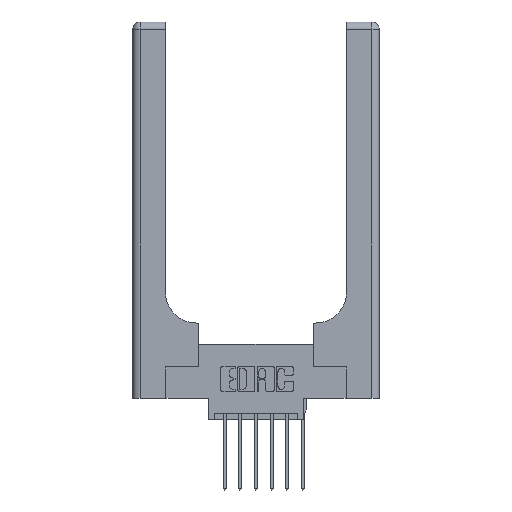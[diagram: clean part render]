
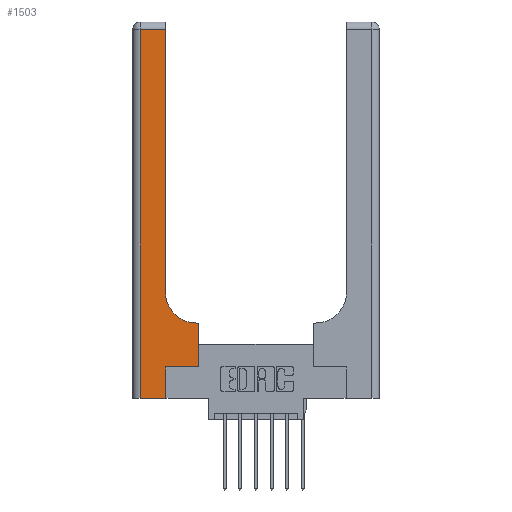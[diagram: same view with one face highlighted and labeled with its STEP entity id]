
A CAD part, top view. The second image highlights one B-rep face of the part: STEP entity #1503.
In plain terms, the highlighted planar face has unit normal (0, 0, 1).
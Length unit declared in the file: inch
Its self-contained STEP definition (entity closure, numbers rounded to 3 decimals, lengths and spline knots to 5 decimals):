
#176 = CARTESIAN_POINT ( 'NONE',  ( 0.26, 0.85, 0.37 ) ) ;
#266 = VECTOR ( 'NONE', #6925, 39.37008 ) ;
#312 = VERTEX_POINT ( 'NONE', #5157 ) ;
#846 = VERTEX_POINT ( 'NONE', #11855 ) ;
#978 = ORIENTED_EDGE ( 'NONE', *, *, #5682, .T. ) ;
#1276 = EDGE_CURVE ( 'NONE', #13701, #12622, #11691, .T. ) ;
#1503 = ADVANCED_FACE ( 'NONE', ( #12878 ), #13950, .F. ) ;
#1708 = DIRECTION ( 'NONE',  ( 1., 0., 0. ) ) ;
#1750 = CIRCLE ( 'NONE', #13360, 0.25 ) ;
#1957 = ORIENTED_EDGE ( 'NONE', *, *, #6541, .T. ) ;
#2016 = CARTESIAN_POINT ( 'NONE',  ( 0.528, 0.25, 0.37 ) ) ;
#2044 = EDGE_CURVE ( 'NONE', #2976, #13701, #1750, .T. ) ;
#2115 = DIRECTION ( 'NONE',  ( -1., 0., 0. ) ) ;
#2976 = VERTEX_POINT ( 'NONE', #3687 ) ;
#3017 = ORIENTED_EDGE ( 'NONE', *, *, #1276, .T. ) ;
#3202 = VECTOR ( 'NONE', #13751, 39.37008 ) ;
#3293 = VERTEX_POINT ( 'NONE', #9776 ) ;
#3356 = DIRECTION ( 'NONE',  ( 1., 0., 0. ) ) ;
#3436 = EDGE_CURVE ( 'NONE', #846, #3293, #11443, .T. ) ;
#3687 = CARTESIAN_POINT ( 'NONE',  ( 0.51, 0.6, 0.37 ) ) ;
#3772 = ORIENTED_EDGE ( 'NONE', *, *, #5378, .T. ) ;
#4036 = EDGE_CURVE ( 'NONE', #3293, #9507, #4855, .T. ) ;
#4099 = DIRECTION ( 'NONE',  ( 1., 0., 0. ) ) ;
#4250 = ORIENTED_EDGE ( 'NONE', *, *, #11842, .T. ) ;
#4713 = LINE ( 'NONE', #5875, #266 ) ;
#4855 = LINE ( 'NONE', #8960, #10240 ) ;
#5157 = CARTESIAN_POINT ( 'NONE',  ( 0.528, 0.25, 0.37 ) ) ;
#5203 = ORIENTED_EDGE ( 'NONE', *, *, #4036, .T. ) ;
#5378 = EDGE_CURVE ( 'NONE', #6536, #2976, #9493, .T. ) ;
#5486 = ORIENTED_EDGE ( 'NONE', *, *, #3436, .T. ) ;
#5620 = EDGE_LOOP ( 'NONE', ( #3017, #978, #13871, #5486, #5203, #1957, #4250, #3772, #9797 ) ) ;
#5682 = EDGE_CURVE ( 'NONE', #12622, #10782, #6336, .T. ) ;
#5688 = VECTOR ( 'NONE', #4099, 39.37008 ) ;
#5775 = DIRECTION ( 'NONE',  ( 0., 1., 0. ) ) ;
#5875 = CARTESIAN_POINT ( 'NONE',  ( 0.06, 3., 0.37 ) ) ;
#6336 = LINE ( 'NONE', #11702, #10401 ) ;
#6536 = VERTEX_POINT ( 'NONE', #13755 ) ;
#6541 = EDGE_CURVE ( 'NONE', #9507, #312, #10551, .T. ) ;
#6819 = VECTOR ( 'NONE', #1708, 39.37008 ) ;
#6925 = DIRECTION ( 'NONE',  ( 0., -1., 0. ) ) ;
#6979 = VECTOR ( 'NONE', #12642, 39.37008 ) ;
#6985 = VECTOR ( 'NONE', #8204, 39.37008 ) ;
#7169 = EDGE_CURVE ( 'NONE', #10782, #846, #4713, .T. ) ;
#7227 = CARTESIAN_POINT ( 'NONE',  ( 0.26, 0.6, 0.37 ) ) ;
#8204 = DIRECTION ( 'NONE',  ( 0., 1., 0. ) ) ;
#8292 = LINE ( 'NONE', #2016, #6979 ) ;
#8744 = CARTESIAN_POINT ( 'NONE',  ( 0.51, 0.85, 0.37 ) ) ;
#8960 = CARTESIAN_POINT ( 'NONE',  ( 0.265, 0., 0.37 ) ) ;
#9493 = LINE ( 'NONE', #7227, #3202 ) ;
#9507 = VERTEX_POINT ( 'NONE', #12911 ) ;
#9594 = CARTESIAN_POINT ( 'NONE',  ( 0.26, 3., 0.37 ) ) ;
#9776 = CARTESIAN_POINT ( 'NONE',  ( 0.265, 0., 0.37 ) ) ;
#9797 = ORIENTED_EDGE ( 'NONE', *, *, #2044, .T. ) ;
#10240 = VECTOR ( 'NONE', #5775, 39.37008 ) ;
#10401 = VECTOR ( 'NONE', #2115, 39.37008 ) ;
#10551 = LINE ( 'NONE', #11819, #5688 ) ;
#10782 = VERTEX_POINT ( 'NONE', #11830 ) ;
#11442 = CARTESIAN_POINT ( 'NONE',  ( 0.26, 2.94, 0.37 ) ) ;
#11443 = LINE ( 'NONE', #11508, #6819 ) ;
#11508 = CARTESIAN_POINT ( 'NONE',  ( 0., 0., 0.37 ) ) ;
#11691 = LINE ( 'NONE', #9594, #6985 ) ;
#11702 = CARTESIAN_POINT ( 'NONE',  ( 0., 2.94, 0.37 ) ) ;
#11795 = CARTESIAN_POINT ( 'NONE',  ( 0., 3., 0.37 ) ) ;
#11819 = CARTESIAN_POINT ( 'NONE',  ( 0.265, 0.25, 0.37 ) ) ;
#11830 = CARTESIAN_POINT ( 'NONE',  ( 0.06, 2.94, 0.37 ) ) ;
#11842 = EDGE_CURVE ( 'NONE', #312, #6536, #8292, .T. ) ;
#11855 = CARTESIAN_POINT ( 'NONE',  ( 0.06, 0., 0.37 ) ) ;
#12072 = DIRECTION ( 'NONE',  ( 0., 0., -1. ) ) ;
#12622 = VERTEX_POINT ( 'NONE', #11442 ) ;
#12642 = DIRECTION ( 'NONE',  ( 0., 1., 0. ) ) ;
#12877 = AXIS2_PLACEMENT_3D ( 'NONE', #11795, #13111, #13882 ) ;
#12878 = FACE_OUTER_BOUND ( 'NONE', #5620, .T. ) ;
#12911 = CARTESIAN_POINT ( 'NONE',  ( 0.265, 0.25, 0.37 ) ) ;
#13111 = DIRECTION ( 'NONE',  ( 0., 0., -1. ) ) ;
#13360 = AXIS2_PLACEMENT_3D ( 'NONE', #8744, #12072, #3356 ) ;
#13701 = VERTEX_POINT ( 'NONE', #176 ) ;
#13751 = DIRECTION ( 'NONE',  ( -1., 0., 0. ) ) ;
#13755 = CARTESIAN_POINT ( 'NONE',  ( 0.528, 0.6, 0.37 ) ) ;
#13871 = ORIENTED_EDGE ( 'NONE', *, *, #7169, .T. ) ;
#13882 = DIRECTION ( 'NONE',  ( -1., 0., 0. ) ) ;
#13950 = PLANE ( 'NONE',  #12877 ) ;
